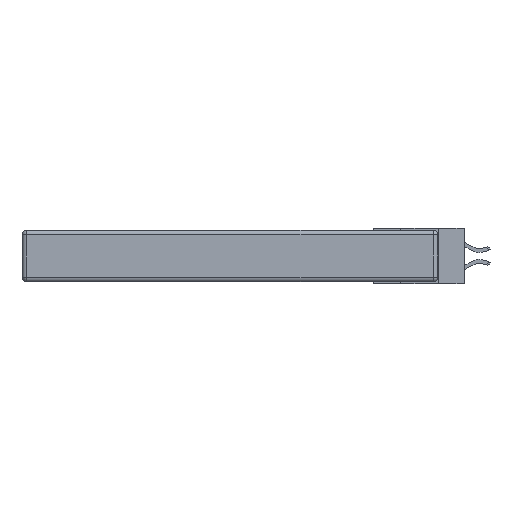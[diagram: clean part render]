
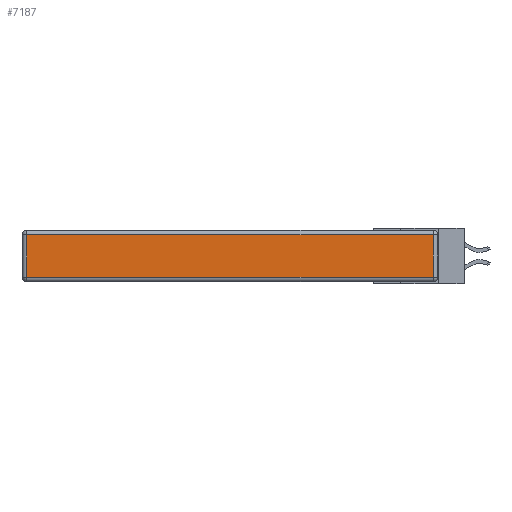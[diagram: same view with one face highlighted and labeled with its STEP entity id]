
A CAD part, left-side view. The second image highlights one B-rep face of the part: STEP entity #7187.
In plain terms, the highlighted planar face has unit normal (-1, 0, 0).
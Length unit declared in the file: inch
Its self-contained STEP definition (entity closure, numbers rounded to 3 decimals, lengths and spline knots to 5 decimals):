
#614 = EDGE_LOOP ( 'NONE', ( #8930, #17508, #6385, #7916 ) ) ;
#2392 = VERTEX_POINT ( 'NONE', #24538 ) ;
#2906 = VERTEX_POINT ( 'NONE', #4631 ) ;
#3389 = VERTEX_POINT ( 'NONE', #15887 ) ;
#4631 = CARTESIAN_POINT ( 'NONE',  ( 0., 2.72, -0.313 ) ) ;
#5069 = CARTESIAN_POINT ( 'NONE',  ( 0., 0., -0.313 ) ) ;
#5117 = LINE ( 'NONE', #17066, #25376 ) ;
#5150 = VERTEX_POINT ( 'NONE', #16485 ) ;
#6385 = ORIENTED_EDGE ( 'NONE', *, *, #25249, .T. ) ;
#7057 = DIRECTION ( 'NONE',  ( 0., 1., 0. ) ) ;
#7187 = ADVANCED_FACE ( 'NONE', ( #15615 ), #18440, .T. ) ;
#7703 = EDGE_CURVE ( 'NONE', #2392, #2906, #11519, .T. ) ;
#7916 = ORIENTED_EDGE ( 'NONE', *, *, #7703, .T. ) ;
#8432 = DIRECTION ( 'NONE',  ( 0., 0., 1. ) ) ;
#8930 = ORIENTED_EDGE ( 'NONE', *, *, #27265, .T. ) ;
#9385 = CARTESIAN_POINT ( 'NONE',  ( 0., 0., -0.343 ) ) ;
#9818 = VECTOR ( 'NONE', #16555, 39.37008 ) ;
#11519 = LINE ( 'NONE', #23244, #9818 ) ;
#11523 = LINE ( 'NONE', #5069, #25013 ) ;
#13844 = DIRECTION ( 'NONE',  ( -1., 0., 0. ) ) ;
#13904 = AXIS2_PLACEMENT_3D ( 'NONE', #9385, #13844, #24502 ) ;
#15615 = FACE_OUTER_BOUND ( 'NONE', #614, .T. ) ;
#15887 = CARTESIAN_POINT ( 'NONE',  ( 0., 0.03, -0.313 ) ) ;
#16412 = VECTOR ( 'NONE', #7057, 39.37008 ) ;
#16485 = CARTESIAN_POINT ( 'NONE',  ( 0., 0.03, -0.03 ) ) ;
#16555 = DIRECTION ( 'NONE',  ( 0., 0., -1. ) ) ;
#17066 = CARTESIAN_POINT ( 'NONE',  ( 0., 0.03, -0.343 ) ) ;
#17508 = ORIENTED_EDGE ( 'NONE', *, *, #21871, .T. ) ;
#17733 = LINE ( 'NONE', #26285, #16412 ) ;
#18440 = PLANE ( 'NONE',  #13904 ) ;
#21871 = EDGE_CURVE ( 'NONE', #3389, #5150, #5117, .T. ) ;
#23244 = CARTESIAN_POINT ( 'NONE',  ( 0., 2.72, -0.343 ) ) ;
#24502 = DIRECTION ( 'NONE',  ( 0., 0., 1. ) ) ;
#24538 = CARTESIAN_POINT ( 'NONE',  ( 0., 2.72, -0.03 ) ) ;
#24721 = DIRECTION ( 'NONE',  ( 0., -1., 0. ) ) ;
#25013 = VECTOR ( 'NONE', #24721, 39.37008 ) ;
#25249 = EDGE_CURVE ( 'NONE', #5150, #2392, #17733, .T. ) ;
#25376 = VECTOR ( 'NONE', #8432, 39.37008 ) ;
#26285 = CARTESIAN_POINT ( 'NONE',  ( 0., 2.75, -0.03 ) ) ;
#27265 = EDGE_CURVE ( 'NONE', #2906, #3389, #11523, .T. ) ;
